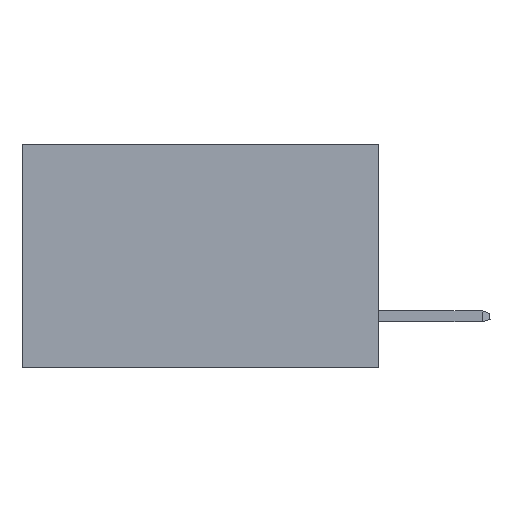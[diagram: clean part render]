
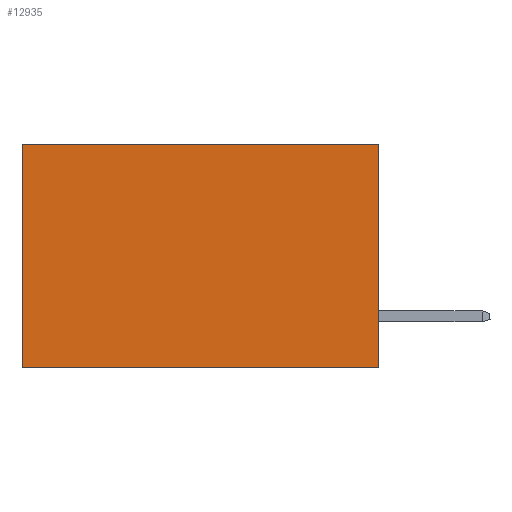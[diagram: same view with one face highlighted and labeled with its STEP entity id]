
A CAD part, left-side view. The second image highlights one B-rep face of the part: STEP entity #12935.
In plain terms, the highlighted planar face has unit normal (-1, 0, 0).
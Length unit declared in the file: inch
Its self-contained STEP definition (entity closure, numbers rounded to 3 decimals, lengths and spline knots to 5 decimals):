
#539 = VECTOR ( 'NONE', #1025, 39.37008 ) ;
#592 = DIRECTION ( 'NONE',  ( 0., 0., -1. ) ) ;
#938 = ORIENTED_EDGE ( 'NONE', *, *, #6142, .F. ) ;
#1025 = DIRECTION ( 'NONE',  ( 0., 1., 0. ) ) ;
#1824 = VERTEX_POINT ( 'NONE', #6843 ) ;
#1913 = VERTEX_POINT ( 'NONE', #10069 ) ;
#2312 = EDGE_CURVE ( 'NONE', #11493, #1824, #11340, .T. ) ;
#2947 = DIRECTION ( 'NONE',  ( 0., 0., -1. ) ) ;
#4005 = CARTESIAN_POINT ( 'NONE',  ( 0.277, 0., -0.37 ) ) ;
#4041 = LINE ( 'NONE', #10718, #12156 ) ;
#6142 = EDGE_CURVE ( 'NONE', #11493, #9504, #8880, .T. ) ;
#6194 = VECTOR ( 'NONE', #11834, 39.37008 ) ;
#6731 = CARTESIAN_POINT ( 'NONE',  ( 0.277, 0., -0.37 ) ) ;
#6843 = CARTESIAN_POINT ( 'NONE',  ( 0.277, 0.59, 0. ) ) ;
#7411 = DIRECTION ( 'NONE',  ( 1., 0., 0. ) ) ;
#7517 = EDGE_LOOP ( 'NONE', ( #9576, #12450, #938, #12768 ) ) ;
#8078 = DIRECTION ( 'NONE',  ( 0., 0., -1. ) ) ;
#8256 = CARTESIAN_POINT ( 'NONE',  ( 0.277, 0., -0.37 ) ) ;
#8272 = EDGE_CURVE ( 'NONE', #1824, #1913, #4041, .T. ) ;
#8713 = CARTESIAN_POINT ( 'NONE',  ( 0.277, 0., -0.37 ) ) ;
#8880 = LINE ( 'NONE', #8256, #11750 ) ;
#9504 = VERTEX_POINT ( 'NONE', #8713 ) ;
#9576 = ORIENTED_EDGE ( 'NONE', *, *, #8272, .T. ) ;
#10069 = CARTESIAN_POINT ( 'NONE',  ( 0.277, 0.59, -0.37 ) ) ;
#10097 = CARTESIAN_POINT ( 'NONE',  ( 0.277, 0., 0. ) ) ;
#10718 = CARTESIAN_POINT ( 'NONE',  ( 0.277, 0.59, -0.37 ) ) ;
#11340 = LINE ( 'NONE', #12247, #6194 ) ;
#11427 = EDGE_CURVE ( 'NONE', #9504, #1913, #12406, .T. ) ;
#11493 = VERTEX_POINT ( 'NONE', #10097 ) ;
#11750 = VECTOR ( 'NONE', #8078, 39.37008 ) ;
#11834 = DIRECTION ( 'NONE',  ( 0., 1., 0. ) ) ;
#12156 = VECTOR ( 'NONE', #2947, 39.37008 ) ;
#12247 = CARTESIAN_POINT ( 'NONE',  ( 0.277, 0., 0. ) ) ;
#12406 = LINE ( 'NONE', #6731, #539 ) ;
#12450 = ORIENTED_EDGE ( 'NONE', *, *, #11427, .F. ) ;
#12768 = ORIENTED_EDGE ( 'NONE', *, *, #2312, .T. ) ;
#12808 = AXIS2_PLACEMENT_3D ( 'NONE', #4005, #7411, #592 ) ;
#12935 = ADVANCED_FACE ( 'NONE', ( #13920 ), #13787, .F. ) ;
#13787 = PLANE ( 'NONE',  #12808 ) ;
#13920 = FACE_OUTER_BOUND ( 'NONE', #7517, .T. ) ;
